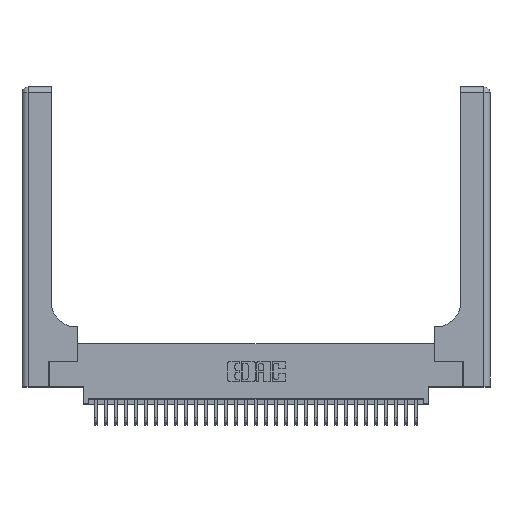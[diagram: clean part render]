
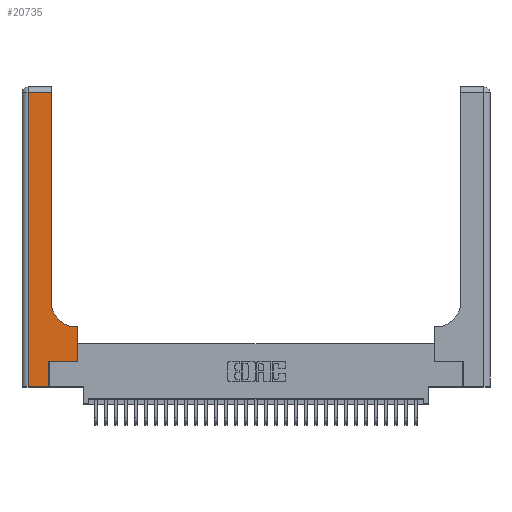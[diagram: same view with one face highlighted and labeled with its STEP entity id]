
A CAD part, top view. The second image highlights one B-rep face of the part: STEP entity #20735.
In plain terms, the highlighted planar face has unit normal (0, 0, 1).
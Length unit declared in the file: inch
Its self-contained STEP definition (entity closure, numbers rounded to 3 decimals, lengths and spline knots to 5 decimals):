
#206 = ORIENTED_EDGE ( 'NONE', *, *, #16445, .T. ) ;
#1065 = EDGE_CURVE ( 'NONE', #7001, #6568, #11460, .T. ) ;
#1479 = DIRECTION ( 'NONE',  ( -1., 0., 0. ) ) ;
#2435 = PLANE ( 'NONE',  #12724 ) ;
#3104 = CARTESIAN_POINT ( 'NONE',  ( 0.2915, 0.85, 0.37 ) ) ;
#3119 = VECTOR ( 'NONE', #22933, 39.37008 ) ;
#3755 = VERTEX_POINT ( 'NONE', #29403 ) ;
#3918 = CARTESIAN_POINT ( 'NONE',  ( 0.269, 0.25, 0.37 ) ) ;
#4672 = EDGE_CURVE ( 'NONE', #33646, #17692, #11705, .T. ) ;
#4716 = CARTESIAN_POINT ( 'NONE',  ( 0.269, 0.25, 0.37 ) ) ;
#4729 = EDGE_CURVE ( 'NONE', #6568, #18123, #31938, .T. ) ;
#5268 = CARTESIAN_POINT ( 'NONE',  ( 0., 2.94, 0.37 ) ) ;
#6132 = CARTESIAN_POINT ( 'NONE',  ( 0.2915, 2.94, 0.37 ) ) ;
#6158 = VECTOR ( 'NONE', #1479, 39.37008 ) ;
#6225 = ORIENTED_EDGE ( 'NONE', *, *, #8440, .T. ) ;
#6568 = VERTEX_POINT ( 'NONE', #11109 ) ;
#6980 = DIRECTION ( 'NONE',  ( 0., -1., 0. ) ) ;
#7001 = VERTEX_POINT ( 'NONE', #3918 ) ;
#7056 = LINE ( 'NONE', #11997, #19814 ) ;
#7181 = CARTESIAN_POINT ( 'NONE',  ( 0.06, 0., 0.37 ) ) ;
#7370 = DIRECTION ( 'NONE',  ( 1., 0., 0. ) ) ;
#7617 = VECTOR ( 'NONE', #17623, 39.37008 ) ;
#7801 = LINE ( 'NONE', #30137, #6158 ) ;
#8157 = DIRECTION ( 'NONE',  ( -1., 0., 0. ) ) ;
#8440 = EDGE_CURVE ( 'NONE', #15954, #7001, #12585, .T. ) ;
#8681 = ORIENTED_EDGE ( 'NONE', *, *, #4672, .T. ) ;
#9607 = DIRECTION ( 'NONE',  ( 0., 1., 0. ) ) ;
#9700 = DIRECTION ( 'NONE',  ( 0., 0., -1. ) ) ;
#10951 = ORIENTED_EDGE ( 'NONE', *, *, #1065, .T. ) ;
#11063 = VECTOR ( 'NONE', #7370, 39.37008 ) ;
#11109 = CARTESIAN_POINT ( 'NONE',  ( 0.5585, 0.25, 0.37 ) ) ;
#11460 = LINE ( 'NONE', #4716, #11063 ) ;
#11461 = ORIENTED_EDGE ( 'NONE', *, *, #22332, .T. ) ;
#11705 = LINE ( 'NONE', #30926, #7617 ) ;
#11754 = DIRECTION ( 'NONE',  ( 0., 1., 0. ) ) ;
#11997 = CARTESIAN_POINT ( 'NONE',  ( 0.06, 3., 0.37 ) ) ;
#12224 = CARTESIAN_POINT ( 'NONE',  ( 0.5415, 0.85, 0.37 ) ) ;
#12585 = LINE ( 'NONE', #22528, #20052 ) ;
#12724 = AXIS2_PLACEMENT_3D ( 'NONE', #31467, #31689, #8157 ) ;
#15349 = EDGE_CURVE ( 'NONE', #3755, #33266, #7056, .T. ) ;
#15826 = AXIS2_PLACEMENT_3D ( 'NONE', #12224, #9700, #20206 ) ;
#15954 = VERTEX_POINT ( 'NONE', #29779 ) ;
#16445 = EDGE_CURVE ( 'NONE', #18123, #19080, #7801, .T. ) ;
#17024 = EDGE_CURVE ( 'NONE', #17692, #3755, #26675, .T. ) ;
#17462 = ORIENTED_EDGE ( 'NONE', *, *, #23894, .T. ) ;
#17623 = DIRECTION ( 'NONE',  ( 0., 1., 0. ) ) ;
#17692 = VERTEX_POINT ( 'NONE', #6132 ) ;
#18123 = VERTEX_POINT ( 'NONE', #34055 ) ;
#19080 = VERTEX_POINT ( 'NONE', #25694 ) ;
#19814 = VECTOR ( 'NONE', #6980, 39.37008 ) ;
#20052 = VECTOR ( 'NONE', #9607, 39.37008 ) ;
#20206 = DIRECTION ( 'NONE',  ( 1., 0., 0. ) ) ;
#20445 = LINE ( 'NONE', #28096, #3119 ) ;
#20735 = ADVANCED_FACE ( 'NONE', ( #31861 ), #2435, .F. ) ;
#22332 = EDGE_CURVE ( 'NONE', #33266, #15954, #20445, .T. ) ;
#22528 = CARTESIAN_POINT ( 'NONE',  ( 0.269, 0., 0.37 ) ) ;
#22933 = DIRECTION ( 'NONE',  ( 1., 0., 0. ) ) ;
#23334 = DIRECTION ( 'NONE',  ( -1., 0., 0. ) ) ;
#23894 = EDGE_CURVE ( 'NONE', #19080, #33646, #31524, .T. ) ;
#24060 = VECTOR ( 'NONE', #11754, 39.37008 ) ;
#24196 = VECTOR ( 'NONE', #23334, 39.37008 ) ;
#25694 = CARTESIAN_POINT ( 'NONE',  ( 0.5415, 0.6, 0.37 ) ) ;
#26675 = LINE ( 'NONE', #5268, #24196 ) ;
#27552 = CARTESIAN_POINT ( 'NONE',  ( 0.5585, 0.25, 0.37 ) ) ;
#28096 = CARTESIAN_POINT ( 'NONE',  ( 0., 0., 0.37 ) ) ;
#28187 = ORIENTED_EDGE ( 'NONE', *, *, #15349, .T. ) ;
#29295 = EDGE_LOOP ( 'NONE', ( #8681, #31109, #28187, #11461, #6225, #10951, #31511, #206, #17462 ) ) ;
#29403 = CARTESIAN_POINT ( 'NONE',  ( 0.06, 2.94, 0.37 ) ) ;
#29779 = CARTESIAN_POINT ( 'NONE',  ( 0.269, 0., 0.37 ) ) ;
#30137 = CARTESIAN_POINT ( 'NONE',  ( 0.2915, 0.6, 0.37 ) ) ;
#30926 = CARTESIAN_POINT ( 'NONE',  ( 0.2915, 3., 0.37 ) ) ;
#31109 = ORIENTED_EDGE ( 'NONE', *, *, #17024, .T. ) ;
#31467 = CARTESIAN_POINT ( 'NONE',  ( 0., 3., 0.37 ) ) ;
#31511 = ORIENTED_EDGE ( 'NONE', *, *, #4729, .T. ) ;
#31524 = CIRCLE ( 'NONE', #15826, 0.25 ) ;
#31689 = DIRECTION ( 'NONE',  ( 0., 0., -1. ) ) ;
#31861 = FACE_OUTER_BOUND ( 'NONE', #29295, .T. ) ;
#31938 = LINE ( 'NONE', #27552, #24060 ) ;
#33266 = VERTEX_POINT ( 'NONE', #7181 ) ;
#33646 = VERTEX_POINT ( 'NONE', #3104 ) ;
#34055 = CARTESIAN_POINT ( 'NONE',  ( 0.5585, 0.6, 0.37 ) ) ;
